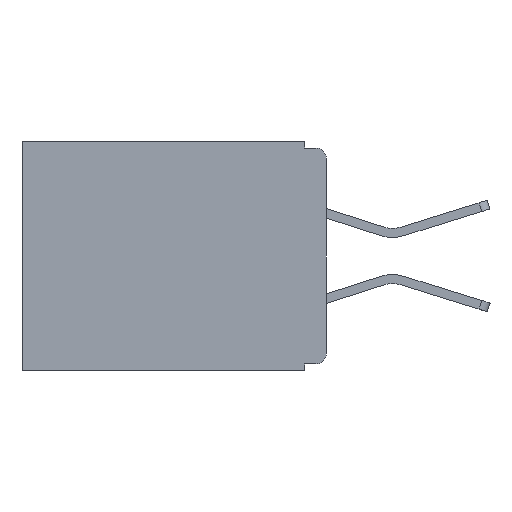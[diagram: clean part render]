
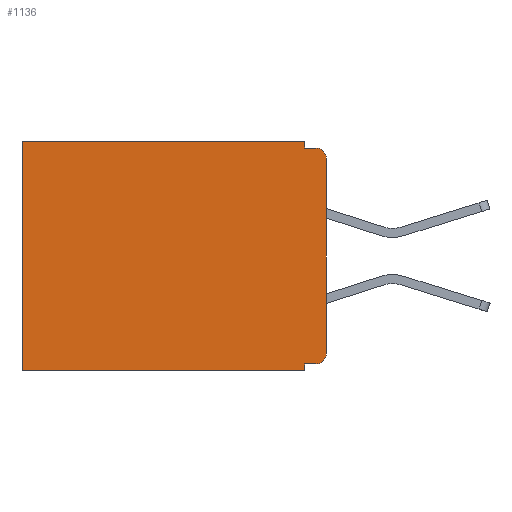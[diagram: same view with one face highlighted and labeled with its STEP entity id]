
A CAD part, left-side view. The second image highlights one B-rep face of the part: STEP entity #1136.
In plain terms, the highlighted planar face has unit normal (-1, 0, 0).
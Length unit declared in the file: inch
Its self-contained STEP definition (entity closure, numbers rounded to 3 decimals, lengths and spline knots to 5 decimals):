
#2 = DIRECTION ( 'NONE',  ( 0., 0., -1. ) ) ;
#289 = VERTEX_POINT ( 'NONE', #2629 ) ;
#649 = CIRCLE ( 'NONE', #7630, 0.015 ) ;
#891 = VECTOR ( 'NONE', #12051, 39.37008 ) ;
#1136 = ADVANCED_FACE ( 'NONE', ( #2085 ), #2248, .F. ) ;
#1280 = EDGE_CURVE ( 'NONE', #4643, #4152, #7872, .T. ) ;
#1451 = ORIENTED_EDGE ( 'NONE', *, *, #6359, .T. ) ;
#1565 = VERTEX_POINT ( 'NONE', #12792 ) ;
#1860 = VERTEX_POINT ( 'NONE', #10381 ) ;
#1961 = EDGE_CURVE ( 'NONE', #4643, #15591, #15482, .T. ) ;
#2003 = CARTESIAN_POINT ( 'NONE',  ( 0.3, 0., -0.32 ) ) ;
#2017 = DIRECTION ( 'NONE',  ( 0., 1., 0. ) ) ;
#2085 = FACE_OUTER_BOUND ( 'NONE', #4384, .T. ) ;
#2173 = DIRECTION ( 'NONE',  ( 1., 0., 0. ) ) ;
#2248 = PLANE ( 'NONE',  #18526 ) ;
#2268 = DIRECTION ( 'NONE',  ( 0., 0., -1. ) ) ;
#2352 = CARTESIAN_POINT ( 'NONE',  ( 0.3, 0.015, -0.305 ) ) ;
#2629 = CARTESIAN_POINT ( 'NONE',  ( 0.3, 0.015, -0.32 ) ) ;
#3056 = LINE ( 'NONE', #5182, #10616 ) ;
#3945 = DIRECTION ( 'NONE',  ( 0., 0., -1. ) ) ;
#4127 = CARTESIAN_POINT ( 'NONE',  ( 0.3, 0., -0.01 ) ) ;
#4152 = VERTEX_POINT ( 'NONE', #10816 ) ;
#4384 = EDGE_LOOP ( 'NONE', ( #16128, #19049, #18069, #4837, #12841, #1451, #9418, #12615, #13495, #10296 ) ) ;
#4480 = EDGE_CURVE ( 'NONE', #289, #5077, #13496, .T. ) ;
#4529 = VECTOR ( 'NONE', #2268, 39.37008 ) ;
#4643 = VERTEX_POINT ( 'NONE', #6272 ) ;
#4837 = ORIENTED_EDGE ( 'NONE', *, *, #9381, .F. ) ;
#5077 = VERTEX_POINT ( 'NONE', #16889 ) ;
#5165 = LINE ( 'NONE', #14046, #12621 ) ;
#5182 = CARTESIAN_POINT ( 'NONE',  ( 0.3, 0.031, -0.33 ) ) ;
#5294 = AXIS2_PLACEMENT_3D ( 'NONE', #17209, #17265, #5740 ) ;
#5614 = VECTOR ( 'NONE', #2, 39.37008 ) ;
#5740 = DIRECTION ( 'NONE',  ( 0., 0., -1. ) ) ;
#5903 = VERTEX_POINT ( 'NONE', #17999 ) ;
#6272 = CARTESIAN_POINT ( 'NONE',  ( 0.3, 0., -0.025 ) ) ;
#6359 = EDGE_CURVE ( 'NONE', #17533, #10174, #8095, .T. ) ;
#6400 = EDGE_CURVE ( 'NONE', #5077, #1565, #3056, .T. ) ;
#6592 = DIRECTION ( 'NONE',  ( 0., 0., -1. ) ) ;
#6659 = CARTESIAN_POINT ( 'NONE',  ( 0.3, 0., 0. ) ) ;
#7630 = AXIS2_PLACEMENT_3D ( 'NONE', #2352, #12930, #3945 ) ;
#7732 = CARTESIAN_POINT ( 'NONE',  ( 0.3, 0.031, 0. ) ) ;
#7872 = CIRCLE ( 'NONE', #5294, 0.015 ) ;
#8095 = LINE ( 'NONE', #18352, #15921 ) ;
#8632 = DIRECTION ( 'NONE',  ( 0., -1., 0. ) ) ;
#9217 = CARTESIAN_POINT ( 'NONE',  ( 0.3, 0., -0.305 ) ) ;
#9381 = EDGE_CURVE ( 'NONE', #5903, #1860, #13521, .T. ) ;
#9418 = ORIENTED_EDGE ( 'NONE', *, *, #16292, .F. ) ;
#9947 = VECTOR ( 'NONE', #8632, 39.37008 ) ;
#10174 = VERTEX_POINT ( 'NONE', #15508 ) ;
#10296 = ORIENTED_EDGE ( 'NONE', *, *, #17767, .T. ) ;
#10381 = CARTESIAN_POINT ( 'NONE',  ( 0.3, 0.031, -0.01 ) ) ;
#10474 = CARTESIAN_POINT ( 'NONE',  ( 0.3, 0., -0.33 ) ) ;
#10616 = VECTOR ( 'NONE', #14088, 39.37008 ) ;
#10622 = VECTOR ( 'NONE', #2017, 39.37008 ) ;
#10816 = CARTESIAN_POINT ( 'NONE',  ( 0.3, 0.015, -0.01 ) ) ;
#11053 = DIRECTION ( 'NONE',  ( 0., 1., 0. ) ) ;
#12051 = DIRECTION ( 'NONE',  ( 0., 1., 0. ) ) ;
#12615 = ORIENTED_EDGE ( 'NONE', *, *, #6400, .F. ) ;
#12621 = VECTOR ( 'NONE', #11053, 39.37008 ) ;
#12792 = CARTESIAN_POINT ( 'NONE',  ( 0.3, 0.031, -0.33 ) ) ;
#12841 = ORIENTED_EDGE ( 'NONE', *, *, #19388, .T. ) ;
#12930 = DIRECTION ( 'NONE',  ( -1., 0., 0. ) ) ;
#13495 = ORIENTED_EDGE ( 'NONE', *, *, #4480, .F. ) ;
#13496 = LINE ( 'NONE', #2003, #891 ) ;
#13502 = EDGE_CURVE ( 'NONE', #1860, #4152, #14363, .T. ) ;
#13521 = LINE ( 'NONE', #7732, #5614 ) ;
#13936 = CARTESIAN_POINT ( 'NONE',  ( 0.3, 0.437, 0. ) ) ;
#14046 = CARTESIAN_POINT ( 'NONE',  ( 0.3, 0., -0.33 ) ) ;
#14088 = DIRECTION ( 'NONE',  ( 0., 0., -1. ) ) ;
#14363 = LINE ( 'NONE', #4127, #9947 ) ;
#14561 = LINE ( 'NONE', #6659, #10622 ) ;
#15157 = CARTESIAN_POINT ( 'NONE',  ( 0.3, 0., -0.33 ) ) ;
#15482 = LINE ( 'NONE', #15157, #4529 ) ;
#15508 = CARTESIAN_POINT ( 'NONE',  ( 0.3, 0.437, -0.33 ) ) ;
#15591 = VERTEX_POINT ( 'NONE', #9217 ) ;
#15921 = VECTOR ( 'NONE', #6592, 39.37008 ) ;
#16128 = ORIENTED_EDGE ( 'NONE', *, *, #1961, .F. ) ;
#16292 = EDGE_CURVE ( 'NONE', #1565, #10174, #5165, .T. ) ;
#16712 = DIRECTION ( 'NONE',  ( 0., 0., -1. ) ) ;
#16889 = CARTESIAN_POINT ( 'NONE',  ( 0.3, 0.031, -0.32 ) ) ;
#17209 = CARTESIAN_POINT ( 'NONE',  ( 0.3, 0.015, -0.025 ) ) ;
#17265 = DIRECTION ( 'NONE',  ( -1., 0., 0. ) ) ;
#17533 = VERTEX_POINT ( 'NONE', #13936 ) ;
#17767 = EDGE_CURVE ( 'NONE', #289, #15591, #649, .T. ) ;
#17999 = CARTESIAN_POINT ( 'NONE',  ( 0.3, 0.031, 0. ) ) ;
#18069 = ORIENTED_EDGE ( 'NONE', *, *, #13502, .F. ) ;
#18352 = CARTESIAN_POINT ( 'NONE',  ( 0.3, 0.437, -0.33 ) ) ;
#18526 = AXIS2_PLACEMENT_3D ( 'NONE', #10474, #2173, #16712 ) ;
#19049 = ORIENTED_EDGE ( 'NONE', *, *, #1280, .T. ) ;
#19388 = EDGE_CURVE ( 'NONE', #5903, #17533, #14561, .T. ) ;
